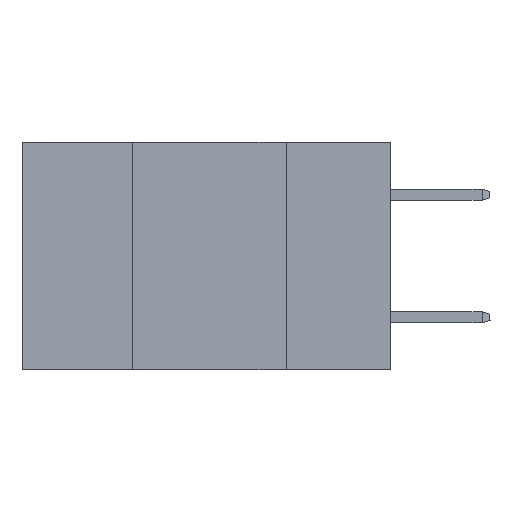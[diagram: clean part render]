
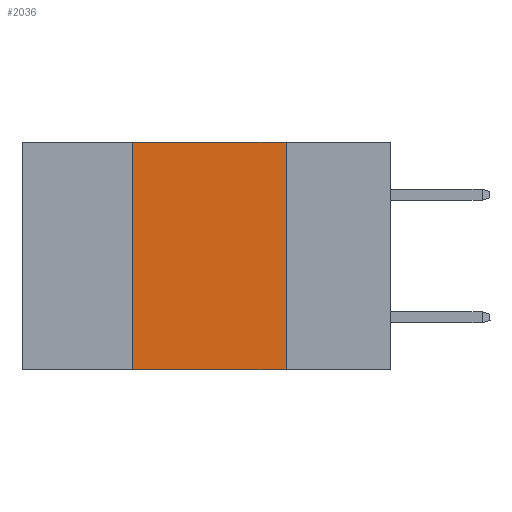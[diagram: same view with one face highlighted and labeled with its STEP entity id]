
A CAD part, left-side view. The second image highlights one B-rep face of the part: STEP entity #2036.
In plain terms, the highlighted planar face has unit normal (-1, 0, 0).
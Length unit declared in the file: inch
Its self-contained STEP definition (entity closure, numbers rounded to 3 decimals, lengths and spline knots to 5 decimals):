
#524 = VERTEX_POINT ( 'NONE', #6446 ) ;
#722 = VERTEX_POINT ( 'NONE', #873 ) ;
#826 = VECTOR ( 'NONE', #8076, 39.37008 ) ;
#873 = CARTESIAN_POINT ( 'NONE',  ( 0., 0.42, 0. ) ) ;
#1300 = LINE ( 'NONE', #9254, #10693 ) ;
#1340 = CARTESIAN_POINT ( 'NONE',  ( 0., 0.17, 0. ) ) ;
#1502 = VERTEX_POINT ( 'NONE', #1340 ) ;
#1557 = CARTESIAN_POINT ( 'NONE',  ( 0., 0.6, -0.37 ) ) ;
#2036 = ADVANCED_FACE ( 'NONE', ( #3963 ), #11944, .F. ) ;
#2071 = VERTEX_POINT ( 'NONE', #6786 ) ;
#3313 = ORIENTED_EDGE ( 'NONE', *, *, #11486, .F. ) ;
#3807 = VECTOR ( 'NONE', #5740, 39.37008 ) ;
#3867 = ORIENTED_EDGE ( 'NONE', *, *, #7298, .F. ) ;
#3963 = FACE_OUTER_BOUND ( 'NONE', #5380, .T. ) ;
#3979 = DIRECTION ( 'NONE',  ( 0., 0., -1. ) ) ;
#4398 = LINE ( 'NONE', #9373, #3807 ) ;
#5268 = EDGE_CURVE ( 'NONE', #524, #2071, #5632, .T. ) ;
#5380 = EDGE_LOOP ( 'NONE', ( #3867, #11569, #3313, #6747 ) ) ;
#5632 = LINE ( 'NONE', #1557, #826 ) ;
#5740 = DIRECTION ( 'NONE',  ( 0., -1., 0. ) ) ;
#5863 = LINE ( 'NONE', #7021, #8559 ) ;
#6446 = CARTESIAN_POINT ( 'NONE',  ( 0., 0.42, -0.37 ) ) ;
#6481 = DIRECTION ( 'NONE',  ( 1., 0., 0. ) ) ;
#6747 = ORIENTED_EDGE ( 'NONE', *, *, #5268, .T. ) ;
#6786 = CARTESIAN_POINT ( 'NONE',  ( 0., 0.17, -0.37 ) ) ;
#7021 = CARTESIAN_POINT ( 'NONE',  ( 0., 0.17, 0. ) ) ;
#7298 = EDGE_CURVE ( 'NONE', #1502, #2071, #5863, .T. ) ;
#8076 = DIRECTION ( 'NONE',  ( 0., -1., 0. ) ) ;
#8559 = VECTOR ( 'NONE', #8840, 39.37008 ) ;
#8658 = AXIS2_PLACEMENT_3D ( 'NONE', #11983, #6481, #3979 ) ;
#8840 = DIRECTION ( 'NONE',  ( 0., 0., -1. ) ) ;
#8967 = EDGE_CURVE ( 'NONE', #722, #1502, #4398, .T. ) ;
#9254 = CARTESIAN_POINT ( 'NONE',  ( 0., 0.42, 0. ) ) ;
#9373 = CARTESIAN_POINT ( 'NONE',  ( 0., 0.6, 0. ) ) ;
#10693 = VECTOR ( 'NONE', #11154, 39.37008 ) ;
#11154 = DIRECTION ( 'NONE',  ( 0., 0., 1. ) ) ;
#11486 = EDGE_CURVE ( 'NONE', #524, #722, #1300, .T. ) ;
#11569 = ORIENTED_EDGE ( 'NONE', *, *, #8967, .F. ) ;
#11944 = PLANE ( 'NONE',  #8658 ) ;
#11983 = CARTESIAN_POINT ( 'NONE',  ( 0., 0.6, 0. ) ) ;
